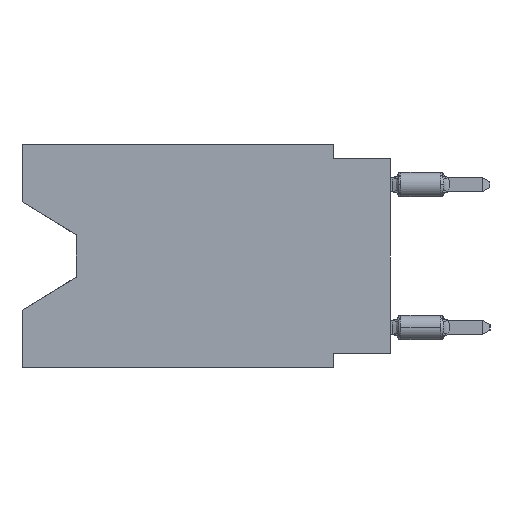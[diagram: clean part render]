
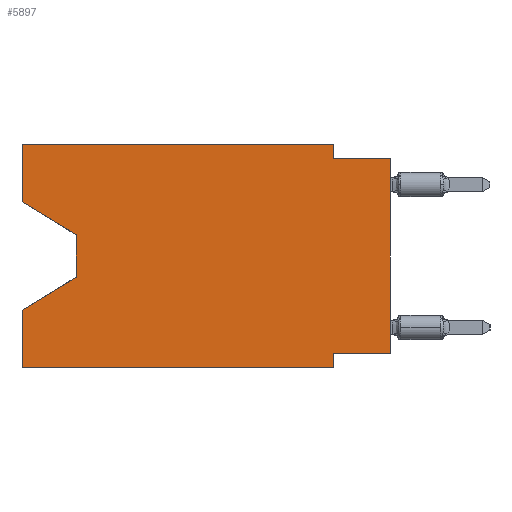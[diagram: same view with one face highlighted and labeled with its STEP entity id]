
A CAD part, left-side view. The second image highlights one B-rep face of the part: STEP entity #5897.
In plain terms, the highlighted planar face has unit normal (-1, 0, 0).
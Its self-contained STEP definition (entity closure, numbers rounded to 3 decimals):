
#419 = LINE ( 'NONE', #13398, #20325 ) ;
#626 = VECTOR ( 'NONE', #22043, 1000. ) ;
#793 = EDGE_CURVE ( 'NONE', #8829, #28922, #3528, .T. ) ;
#1097 = CARTESIAN_POINT ( 'NONE',  ( 0., 13.97, -5.893 ) ) ;
#1347 = VECTOR ( 'NONE', #26558, 1000. ) ;
#1349 = EDGE_CURVE ( 'NONE', #31336, #22022, #16981, .T. ) ;
#1948 = EDGE_CURVE ( 'NONE', #25405, #8469, #12542, .T. ) ;
#2157 = CARTESIAN_POINT ( 'NONE',  ( 0., 13.97, -4.013 ) ) ;
#2664 = ORIENTED_EDGE ( 'NONE', *, *, #11425, .F. ) ;
#2967 = VECTOR ( 'NONE', #33152, 1000. ) ;
#3311 = CARTESIAN_POINT ( 'NONE',  ( 0., 16.383, 0. ) ) ;
#3348 = LINE ( 'NONE', #13905, #1347 ) ;
#3528 = LINE ( 'NONE', #19284, #626 ) ;
#3541 = CARTESIAN_POINT ( 'NONE',  ( 0., 13.97, -4.013 ) ) ;
#4102 = VECTOR ( 'NONE', #29366, 1000. ) ;
#4357 = DIRECTION ( 'NONE',  ( 1., 0., 0. ) ) ;
#4520 = ORIENTED_EDGE ( 'NONE', *, *, #15222, .T. ) ;
#5297 = VERTEX_POINT ( 'NONE', #1097 ) ;
#5668 = CARTESIAN_POINT ( 'NONE',  ( 0., 16.383, -9.906 ) ) ;
#5897 = ADVANCED_FACE ( 'NONE', ( #7315 ), #14916, .F. ) ;
#6700 = CARTESIAN_POINT ( 'NONE',  ( 0., 0., -0.635 ) ) ;
#6807 = VECTOR ( 'NONE', #7207, 1000. ) ;
#7207 = DIRECTION ( 'NONE',  ( 0., 0., -1. ) ) ;
#7315 = FACE_OUTER_BOUND ( 'NONE', #29165, .T. ) ;
#7989 = ORIENTED_EDGE ( 'NONE', *, *, #14146, .F. ) ;
#8469 = VERTEX_POINT ( 'NONE', #9473 ) ;
#8829 = VERTEX_POINT ( 'NONE', #25988 ) ;
#8924 = VECTOR ( 'NONE', #30305, 1000. ) ;
#8984 = VERTEX_POINT ( 'NONE', #30107 ) ;
#9203 = CARTESIAN_POINT ( 'NONE',  ( 0., 16.383, 0. ) ) ;
#9473 = CARTESIAN_POINT ( 'NONE',  ( 0., 2.54, -9.271 ) ) ;
#9952 = CARTESIAN_POINT ( 'NONE',  ( 0., 0., -9.271 ) ) ;
#10185 = ORIENTED_EDGE ( 'NONE', *, *, #13726, .T. ) ;
#10879 = CARTESIAN_POINT ( 'NONE',  ( 0., 2.54, -9.906 ) ) ;
#11235 = VECTOR ( 'NONE', #21275, 1000. ) ;
#11406 = LINE ( 'NONE', #19367, #33071 ) ;
#11412 = CARTESIAN_POINT ( 'NONE',  ( 0., 2.54, 0. ) ) ;
#11425 = EDGE_CURVE ( 'NONE', #8469, #30191, #419, .T. ) ;
#11479 = VERTEX_POINT ( 'NONE', #32072 ) ;
#12002 = LINE ( 'NONE', #30507, #26774 ) ;
#12542 = LINE ( 'NONE', #9952, #15614 ) ;
#12631 = ORIENTED_EDGE ( 'NONE', *, *, #24082, .F. ) ;
#13398 = CARTESIAN_POINT ( 'NONE',  ( 0., 2.54, -9.906 ) ) ;
#13726 = EDGE_CURVE ( 'NONE', #28922, #5297, #20517, .T. ) ;
#13905 = CARTESIAN_POINT ( 'NONE',  ( 0., 0., 0. ) ) ;
#14146 = EDGE_CURVE ( 'NONE', #8829, #31336, #26000, .T. ) ;
#14214 = VERTEX_POINT ( 'NONE', #15286 ) ;
#14640 = ORIENTED_EDGE ( 'NONE', *, *, #32261, .F. ) ;
#14797 = EDGE_CURVE ( 'NONE', #24157, #30191, #18806, .T. ) ;
#14916 = PLANE ( 'NONE',  #14944 ) ;
#14944 = AXIS2_PLACEMENT_3D ( 'NONE', #28231, #4357, #33756 ) ;
#15054 = ORIENTED_EDGE ( 'NONE', *, *, #1948, .F. ) ;
#15062 = ORIENTED_EDGE ( 'NONE', *, *, #1349, .F. ) ;
#15222 = EDGE_CURVE ( 'NONE', #25405, #14214, #3348, .T. ) ;
#15286 = CARTESIAN_POINT ( 'NONE',  ( 0., 0., -0.635 ) ) ;
#15299 = EDGE_CURVE ( 'NONE', #5297, #8984, #12002, .T. ) ;
#15314 = DIRECTION ( 'NONE',  ( 0., 1., 0. ) ) ;
#15614 = VECTOR ( 'NONE', #15314, 1000. ) ;
#16606 = CARTESIAN_POINT ( 'NONE',  ( 0., 0., -9.271 ) ) ;
#16981 = LINE ( 'NONE', #27360, #33801 ) ;
#18806 = LINE ( 'NONE', #5668, #4102 ) ;
#19034 = CARTESIAN_POINT ( 'NONE',  ( 0., 16.383, -9.906 ) ) ;
#19284 = CARTESIAN_POINT ( 'NONE',  ( 0., 16.383, -2.546 ) ) ;
#19367 = CARTESIAN_POINT ( 'NONE',  ( 0., 2.54, 0. ) ) ;
#20325 = VECTOR ( 'NONE', #23964, 1000. ) ;
#20517 = LINE ( 'NONE', #2157, #6807 ) ;
#21275 = DIRECTION ( 'NONE',  ( 0., 0., 1. ) ) ;
#21647 = EDGE_CURVE ( 'NONE', #24157, #8984, #32886, .T. ) ;
#21968 = ORIENTED_EDGE ( 'NONE', *, *, #21647, .F. ) ;
#22022 = VERTEX_POINT ( 'NONE', #11412 ) ;
#22043 = DIRECTION ( 'NONE',  ( 0., -0.855, -0.519 ) ) ;
#22336 = DIRECTION ( 'NONE',  ( 0., -1., 0. ) ) ;
#22901 = CARTESIAN_POINT ( 'NONE',  ( 0., 16.383, 0. ) ) ;
#22963 = LINE ( 'NONE', #6700, #2967 ) ;
#23964 = DIRECTION ( 'NONE',  ( 0., 0., -1. ) ) ;
#24082 = EDGE_CURVE ( 'NONE', #22022, #11479, #11406, .T. ) ;
#24157 = VERTEX_POINT ( 'NONE', #19034 ) ;
#25405 = VERTEX_POINT ( 'NONE', #16606 ) ;
#25988 = CARTESIAN_POINT ( 'NONE',  ( 0., 16.383, -2.546 ) ) ;
#26000 = LINE ( 'NONE', #22901, #11235 ) ;
#26558 = DIRECTION ( 'NONE',  ( 0., 0., 1. ) ) ;
#26774 = VECTOR ( 'NONE', #30335, 1000. ) ;
#27360 = CARTESIAN_POINT ( 'NONE',  ( 0., 16.383, 0. ) ) ;
#28231 = CARTESIAN_POINT ( 'NONE',  ( 0., 16.383, 0. ) ) ;
#28922 = VERTEX_POINT ( 'NONE', #3541 ) ;
#29165 = EDGE_LOOP ( 'NONE', ( #32654, #10185, #33297, #21968, #32933, #2664, #15054, #4520, #14640, #12631, #15062, #7989 ) ) ;
#29366 = DIRECTION ( 'NONE',  ( 0., -1., 0. ) ) ;
#30107 = CARTESIAN_POINT ( 'NONE',  ( 0., 16.383, -7.36 ) ) ;
#30191 = VERTEX_POINT ( 'NONE', #10879 ) ;
#30305 = DIRECTION ( 'NONE',  ( 0., 0., 1. ) ) ;
#30335 = DIRECTION ( 'NONE',  ( 0., 0.855, -0.519 ) ) ;
#30507 = CARTESIAN_POINT ( 'NONE',  ( 0., 13.97, -5.893 ) ) ;
#31336 = VERTEX_POINT ( 'NONE', #3311 ) ;
#31824 = DIRECTION ( 'NONE',  ( 0., 0., -1. ) ) ;
#32072 = CARTESIAN_POINT ( 'NONE',  ( 0., 2.54, -0.635 ) ) ;
#32261 = EDGE_CURVE ( 'NONE', #11479, #14214, #22963, .T. ) ;
#32654 = ORIENTED_EDGE ( 'NONE', *, *, #793, .T. ) ;
#32886 = LINE ( 'NONE', #9203, #8924 ) ;
#32933 = ORIENTED_EDGE ( 'NONE', *, *, #14797, .T. ) ;
#33071 = VECTOR ( 'NONE', #31824, 1000. ) ;
#33152 = DIRECTION ( 'NONE',  ( 0., -1., 0. ) ) ;
#33297 = ORIENTED_EDGE ( 'NONE', *, *, #15299, .T. ) ;
#33756 = DIRECTION ( 'NONE',  ( 0., 0., -1. ) ) ;
#33801 = VECTOR ( 'NONE', #22336, 1000. ) ;
